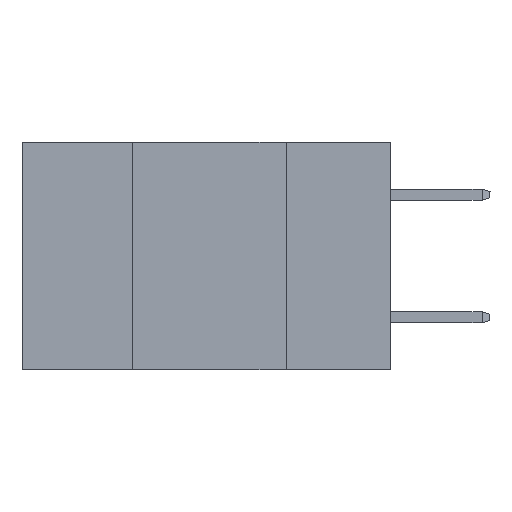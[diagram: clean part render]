
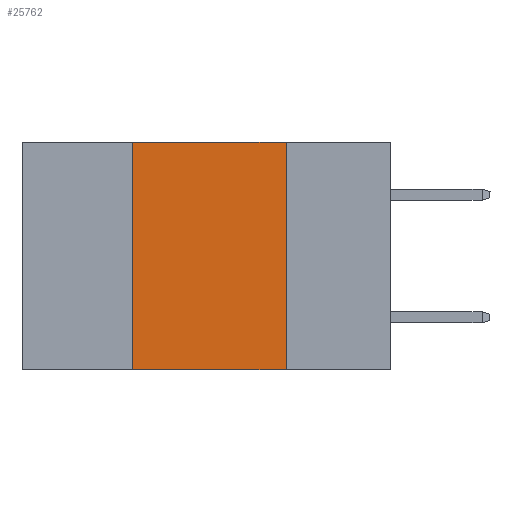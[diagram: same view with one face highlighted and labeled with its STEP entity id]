
A CAD part, left-side view. The second image highlights one B-rep face of the part: STEP entity #25762.
In plain terms, the highlighted planar face has unit normal (-1, 0, 0).
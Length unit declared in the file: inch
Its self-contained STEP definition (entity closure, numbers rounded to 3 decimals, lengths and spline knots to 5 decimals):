
#711 = DIRECTION ( 'NONE',  ( 0., -1., 0. ) ) ;
#1197 = CARTESIAN_POINT ( 'NONE',  ( 0., 0.17, -0.37 ) ) ;
#1367 = AXIS2_PLACEMENT_3D ( 'NONE', #1685, #3852, #18969 ) ;
#1685 = CARTESIAN_POINT ( 'NONE',  ( 0., 0.6, 0. ) ) ;
#3670 = CARTESIAN_POINT ( 'NONE',  ( 0., 0.17, 0. ) ) ;
#3852 = DIRECTION ( 'NONE',  ( 1., 0., 0. ) ) ;
#4129 = LINE ( 'NONE', #20442, #9230 ) ;
#4509 = EDGE_CURVE ( 'NONE', #24449, #21108, #10610, .T. ) ;
#5083 = ORIENTED_EDGE ( 'NONE', *, *, #4509, .T. ) ;
#5237 = VERTEX_POINT ( 'NONE', #17163 ) ;
#5314 = DIRECTION ( 'NONE',  ( 0., 0., 1. ) ) ;
#5489 = EDGE_CURVE ( 'NONE', #5237, #21852, #26346, .T. ) ;
#5843 = DIRECTION ( 'NONE',  ( 0., 0., -1. ) ) ;
#6059 = FACE_OUTER_BOUND ( 'NONE', #19826, .T. ) ;
#7113 = CARTESIAN_POINT ( 'NONE',  ( 0., 0.6, 0. ) ) ;
#7924 = EDGE_CURVE ( 'NONE', #21852, #21108, #16205, .T. ) ;
#9230 = VECTOR ( 'NONE', #5314, 39.37008 ) ;
#10462 = ORIENTED_EDGE ( 'NONE', *, *, #5489, .F. ) ;
#10610 = LINE ( 'NONE', #14930, #26399 ) ;
#12825 = ORIENTED_EDGE ( 'NONE', *, *, #7924, .F. ) ;
#14647 = PLANE ( 'NONE',  #1367 ) ;
#14930 = CARTESIAN_POINT ( 'NONE',  ( 0., 0.6, -0.37 ) ) ;
#15526 = VECTOR ( 'NONE', #5843, 39.37008 ) ;
#16205 = LINE ( 'NONE', #3670, #15526 ) ;
#16288 = EDGE_CURVE ( 'NONE', #24449, #5237, #4129, .T. ) ;
#16897 = ORIENTED_EDGE ( 'NONE', *, *, #16288, .F. ) ;
#17163 = CARTESIAN_POINT ( 'NONE',  ( 0., 0.42, 0. ) ) ;
#18969 = DIRECTION ( 'NONE',  ( 0., 0., -1. ) ) ;
#19251 = DIRECTION ( 'NONE',  ( 0., -1., 0. ) ) ;
#19323 = VECTOR ( 'NONE', #711, 39.37008 ) ;
#19826 = EDGE_LOOP ( 'NONE', ( #12825, #10462, #16897, #5083 ) ) ;
#20442 = CARTESIAN_POINT ( 'NONE',  ( 0., 0.42, 0. ) ) ;
#21108 = VERTEX_POINT ( 'NONE', #1197 ) ;
#21852 = VERTEX_POINT ( 'NONE', #24225 ) ;
#24225 = CARTESIAN_POINT ( 'NONE',  ( 0., 0.17, 0. ) ) ;
#24449 = VERTEX_POINT ( 'NONE', #26451 ) ;
#25762 = ADVANCED_FACE ( 'NONE', ( #6059 ), #14647, .F. ) ;
#26346 = LINE ( 'NONE', #7113, #19323 ) ;
#26399 = VECTOR ( 'NONE', #19251, 39.37008 ) ;
#26451 = CARTESIAN_POINT ( 'NONE',  ( 0., 0.42, -0.37 ) ) ;
